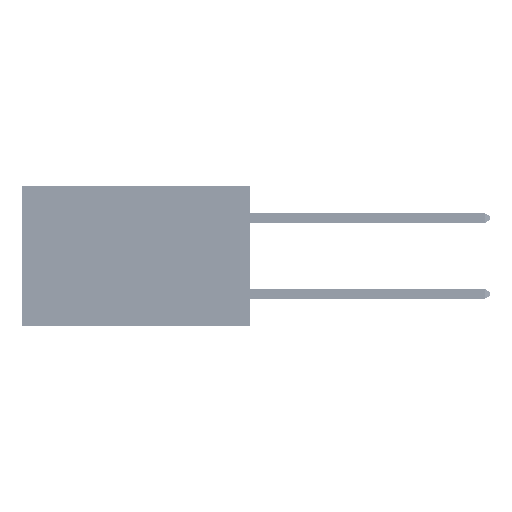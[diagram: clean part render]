
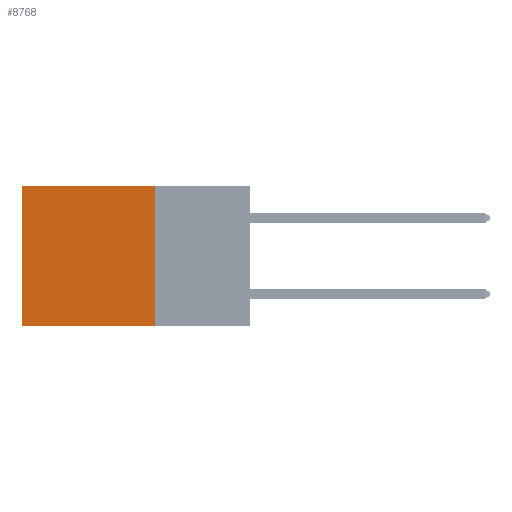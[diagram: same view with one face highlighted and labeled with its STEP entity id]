
A CAD part, left-side view. The second image highlights one B-rep face of the part: STEP entity #8768.
In plain terms, the highlighted planar face has unit normal (-1, 0, 0).
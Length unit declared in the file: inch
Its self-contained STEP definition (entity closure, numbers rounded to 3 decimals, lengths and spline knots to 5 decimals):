
#618 = DIRECTION ( 'NONE',  ( 0., 1., 0. ) ) ;
#1001 = CARTESIAN_POINT ( 'NONE',  ( 0.2875, 0.25, 0. ) ) ;
#1330 = LINE ( 'NONE', #14239, #4813 ) ;
#4588 = DIRECTION ( 'NONE',  ( 1., 0., 0. ) ) ;
#4813 = VECTOR ( 'NONE', #21457, 39.37008 ) ;
#5143 = VERTEX_POINT ( 'NONE', #41647 ) ;
#8105 = AXIS2_PLACEMENT_3D ( 'NONE', #39917, #4588, #32181 ) ;
#8132 = CARTESIAN_POINT ( 'NONE',  ( 0.2875, 0.25, -0.37 ) ) ;
#8768 = ADVANCED_FACE ( 'NONE', ( #28075 ), #24199, .F. ) ;
#10283 = VECTOR ( 'NONE', #618, 39.37008 ) ;
#11288 = VERTEX_POINT ( 'NONE', #42577 ) ;
#13871 = EDGE_CURVE ( 'NONE', #24662, #11288, #32383, .T. ) ;
#14239 = CARTESIAN_POINT ( 'NONE',  ( 0.2875, 0.6, 0. ) ) ;
#19398 = EDGE_CURVE ( 'NONE', #24662, #41490, #40223, .T. ) ;
#21457 = DIRECTION ( 'NONE',  ( 0., 0., -1. ) ) ;
#24199 = PLANE ( 'NONE',  #8105 ) ;
#24662 = VERTEX_POINT ( 'NONE', #38875 ) ;
#26448 = ORIENTED_EDGE ( 'NONE', *, *, #47189, .T. ) ;
#28075 = FACE_OUTER_BOUND ( 'NONE', #42133, .T. ) ;
#28231 = CARTESIAN_POINT ( 'NONE',  ( 0.2875, 0.25, -0.37 ) ) ;
#28935 = ORIENTED_EDGE ( 'NONE', *, *, #13871, .T. ) ;
#32181 = DIRECTION ( 'NONE',  ( 0., 0., -1. ) ) ;
#32383 = LINE ( 'NONE', #45006, #37127 ) ;
#36339 = DIRECTION ( 'NONE',  ( 0., 0., -1. ) ) ;
#37127 = VECTOR ( 'NONE', #44240, 39.37008 ) ;
#38751 = EDGE_CURVE ( 'NONE', #41490, #5143, #43968, .T. ) ;
#38875 = CARTESIAN_POINT ( 'NONE',  ( 0.2875, 0.25, 0. ) ) ;
#39917 = CARTESIAN_POINT ( 'NONE',  ( 0.2875, 0.25, 0. ) ) ;
#40223 = LINE ( 'NONE', #1001, #41251 ) ;
#41251 = VECTOR ( 'NONE', #36339, 39.37008 ) ;
#41490 = VERTEX_POINT ( 'NONE', #28231 ) ;
#41647 = CARTESIAN_POINT ( 'NONE',  ( 0.2875, 0.6, -0.37 ) ) ;
#42133 = EDGE_LOOP ( 'NONE', ( #26448, #43525, #50422, #28935 ) ) ;
#42577 = CARTESIAN_POINT ( 'NONE',  ( 0.2875, 0.6, 0. ) ) ;
#43525 = ORIENTED_EDGE ( 'NONE', *, *, #38751, .F. ) ;
#43968 = LINE ( 'NONE', #8132, #10283 ) ;
#44240 = DIRECTION ( 'NONE',  ( 0., 1., 0. ) ) ;
#45006 = CARTESIAN_POINT ( 'NONE',  ( 0.2875, 0.25, 0. ) ) ;
#47189 = EDGE_CURVE ( 'NONE', #11288, #5143, #1330, .T. ) ;
#50422 = ORIENTED_EDGE ( 'NONE', *, *, #19398, .F. ) ;
